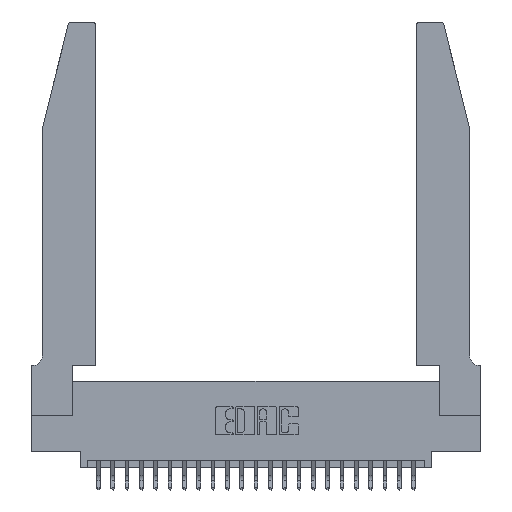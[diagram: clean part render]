
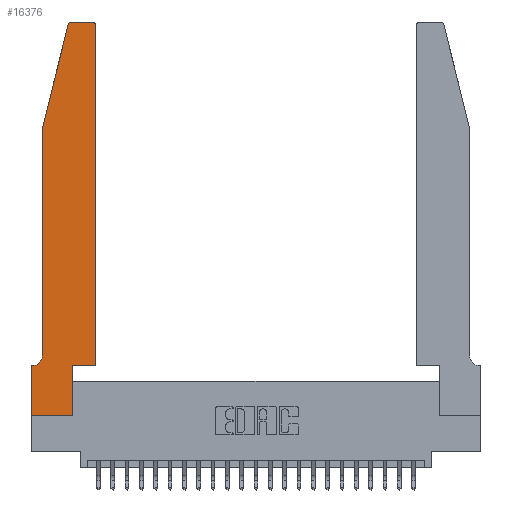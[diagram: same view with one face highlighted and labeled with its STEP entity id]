
A CAD part, top view. The second image highlights one B-rep face of the part: STEP entity #16376.
In plain terms, the highlighted planar face has unit normal (0, 0, 1).
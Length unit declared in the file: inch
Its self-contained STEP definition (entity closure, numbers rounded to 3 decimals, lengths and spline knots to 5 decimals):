
#189 = ORIENTED_EDGE ( 'NONE', *, *, #2360, .T. ) ;
#494 = DIRECTION ( 'NONE',  ( 1., 0., 0. ) ) ;
#630 = LINE ( 'NONE', #22054, #24865 ) ;
#777 = CIRCLE ( 'NONE', #3475, 0.03 ) ;
#1740 = PLANE ( 'NONE',  #3651 ) ;
#1956 = ORIENTED_EDGE ( 'NONE', *, *, #23945, .T. ) ;
#2167 = ORIENTED_EDGE ( 'NONE', *, *, #21607, .T. ) ;
#2360 = EDGE_CURVE ( 'NONE', #24390, #8492, #25150, .T. ) ;
#2530 = LINE ( 'NONE', #25444, #24893 ) ;
#3196 = ORIENTED_EDGE ( 'NONE', *, *, #23025, .T. ) ;
#3216 = DIRECTION ( 'NONE',  ( -1., 0., 0. ) ) ;
#3218 = CARTESIAN_POINT ( 'NONE',  ( 0.0055, 0.35, 0.37 ) ) ;
#3454 = CARTESIAN_POINT ( 'NONE',  ( 0., 0., 0.37 ) ) ;
#3475 = AXIS2_PLACEMENT_3D ( 'NONE', #18984, #17224, #25149 ) ;
#3501 = LINE ( 'NONE', #3454, #16525 ) ;
#3575 = EDGE_LOOP ( 'NONE', ( #5373, #11922, #1956, #13291, #189, #2167, #12911, #5540, #16597, #3196, #10470, #24929 ) ) ;
#3651 = AXIS2_PLACEMENT_3D ( 'NONE', #3890, #12342, #494 ) ;
#3740 = VECTOR ( 'NONE', #5980, 39.37008 ) ;
#3890 = CARTESIAN_POINT ( 'NONE',  ( 0., 0.35, 0.37 ) ) ;
#4422 = DIRECTION ( 'NONE',  ( -1., 0., 0. ) ) ;
#4935 = EDGE_CURVE ( 'NONE', #20659, #11247, #25615, .T. ) ;
#4938 = CARTESIAN_POINT ( 'NONE',  ( 0.284, 2.72, 0.37 ) ) ;
#5136 = VECTOR ( 'NONE', #3216, 39.37008 ) ;
#5190 = CARTESIAN_POINT ( 'NONE',  ( 0.0755, 2., 0.37 ) ) ;
#5373 = ORIENTED_EDGE ( 'NONE', *, *, #4935, .T. ) ;
#5540 = ORIENTED_EDGE ( 'NONE', *, *, #24518, .T. ) ;
#5677 = CARTESIAN_POINT ( 'NONE',  ( 0.25487, 2.72718, 0.37 ) ) ;
#5772 = CARTESIAN_POINT ( 'NONE',  ( 0.4505, 0.35, 0.37 ) ) ;
#5960 = DIRECTION ( 'NONE',  ( 1., 0., 0. ) ) ;
#5980 = DIRECTION ( 'NONE',  ( 0., 1., 0. ) ) ;
#6616 = CARTESIAN_POINT ( 'NONE',  ( 0.0055, 0.42, 0.37 ) ) ;
#6850 = VECTOR ( 'NONE', #20127, 39.37008 ) ;
#7548 = DIRECTION ( 'NONE',  ( -0.239, -0.971, 0. ) ) ;
#8492 = VERTEX_POINT ( 'NONE', #3218 ) ;
#9051 = VERTEX_POINT ( 'NONE', #5677 ) ;
#9086 = LINE ( 'NONE', #22399, #25233 ) ;
#9569 = FACE_OUTER_BOUND ( 'NONE', #3575, .T. ) ;
#9613 = CARTESIAN_POINT ( 'NONE',  ( 0.2865, 0., 0.37 ) ) ;
#10096 = DIRECTION ( 'NONE',  ( 0., 1., 0. ) ) ;
#10343 = VERTEX_POINT ( 'NONE', #9613 ) ;
#10346 = DIRECTION ( 'NONE',  ( 1., 0., 0. ) ) ;
#10423 = AXIS2_PLACEMENT_3D ( 'NONE', #6616, #20361, #4422 ) ;
#10454 = CARTESIAN_POINT ( 'NONE',  ( 0.0755, 0.35, 0.37 ) ) ;
#10470 = ORIENTED_EDGE ( 'NONE', *, *, #21304, .T. ) ;
#10614 = CARTESIAN_POINT ( 'NONE',  ( 0.0755, 2., 0.37 ) ) ;
#11247 = VERTEX_POINT ( 'NONE', #11436 ) ;
#11436 = CARTESIAN_POINT ( 'NONE',  ( 0.284, 2.75, 0.37 ) ) ;
#11484 = LINE ( 'NONE', #17834, #3740 ) ;
#11818 = AXIS2_PLACEMENT_3D ( 'NONE', #4938, #13030, #18896 ) ;
#11922 = ORIENTED_EDGE ( 'NONE', *, *, #21630, .T. ) ;
#12044 = LINE ( 'NONE', #10614, #6850 ) ;
#12342 = DIRECTION ( 'NONE',  ( 0., 0., 1. ) ) ;
#12807 = CARTESIAN_POINT ( 'NONE',  ( 0.2605, 2.75, 0.37 ) ) ;
#12911 = ORIENTED_EDGE ( 'NONE', *, *, #22553, .T. ) ;
#13030 = DIRECTION ( 'NONE',  ( 0., 0., 1. ) ) ;
#13127 = DIRECTION ( 'NONE',  ( 0., -1., 0. ) ) ;
#13291 = ORIENTED_EDGE ( 'NONE', *, *, #15593, .T. ) ;
#13425 = CARTESIAN_POINT ( 'NONE',  ( 0.2865, 0.35, 0.37 ) ) ;
#13945 = EDGE_CURVE ( 'NONE', #20660, #20659, #777, .T. ) ;
#13965 = CIRCLE ( 'NONE', #11818, 0.03 ) ;
#15593 = EDGE_CURVE ( 'NONE', #15837, #24390, #12044, .T. ) ;
#15837 = VERTEX_POINT ( 'NONE', #5190 ) ;
#16081 = VERTEX_POINT ( 'NONE', #5772 ) ;
#16376 = ADVANCED_FACE ( 'NONE', ( #9569 ), #1740, .T. ) ;
#16525 = VECTOR ( 'NONE', #13127, 39.37008 ) ;
#16597 = ORIENTED_EDGE ( 'NONE', *, *, #24557, .T. ) ;
#17224 = DIRECTION ( 'NONE',  ( 0., 0., 1. ) ) ;
#17834 = CARTESIAN_POINT ( 'NONE',  ( 0.4505, 0.35, 0.37 ) ) ;
#18896 = DIRECTION ( 'NONE',  ( 1., 0., 0. ) ) ;
#18984 = CARTESIAN_POINT ( 'NONE',  ( 0.4205, 2.72, 0.37 ) ) ;
#20127 = DIRECTION ( 'NONE',  ( 0., -1., 0. ) ) ;
#20361 = DIRECTION ( 'NONE',  ( 0., 0., -1. ) ) ;
#20478 = VERTEX_POINT ( 'NONE', #21208 ) ;
#20659 = VERTEX_POINT ( 'NONE', #21619 ) ;
#20660 = VERTEX_POINT ( 'NONE', #23518 ) ;
#21053 = CARTESIAN_POINT ( 'NONE',  ( 0.0755, 0.42, 0.37 ) ) ;
#21208 = CARTESIAN_POINT ( 'NONE',  ( 0., 0.35, 0.37 ) ) ;
#21226 = CARTESIAN_POINT ( 'NONE',  ( 0., 0., 0.37 ) ) ;
#21304 = EDGE_CURVE ( 'NONE', #16081, #20660, #11484, .T. ) ;
#21607 = EDGE_CURVE ( 'NONE', #8492, #20478, #24181, .T. ) ;
#21619 = CARTESIAN_POINT ( 'NONE',  ( 0.4205, 2.75, 0.37 ) ) ;
#21630 = EDGE_CURVE ( 'NONE', #11247, #9051, #13965, .T. ) ;
#21788 = VERTEX_POINT ( 'NONE', #21226 ) ;
#21979 = CARTESIAN_POINT ( 'NONE',  ( 0.2865, 0.35, 0.37 ) ) ;
#22019 = LINE ( 'NONE', #21979, #25486 ) ;
#22054 = CARTESIAN_POINT ( 'NONE',  ( 0., 0., 0.37 ) ) ;
#22249 = VERTEX_POINT ( 'NONE', #13425 ) ;
#22399 = CARTESIAN_POINT ( 'NONE',  ( 0.4505, 0.35, 0.37 ) ) ;
#22553 = EDGE_CURVE ( 'NONE', #20478, #21788, #3501, .T. ) ;
#23025 = EDGE_CURVE ( 'NONE', #22249, #16081, #9086, .T. ) ;
#23518 = CARTESIAN_POINT ( 'NONE',  ( 0.4505, 2.72, 0.37 ) ) ;
#23945 = EDGE_CURVE ( 'NONE', #9051, #15837, #2530, .T. ) ;
#24132 = VECTOR ( 'NONE', #24339, 39.37008 ) ;
#24181 = LINE ( 'NONE', #10454, #24132 ) ;
#24339 = DIRECTION ( 'NONE',  ( -1., 0., 0. ) ) ;
#24390 = VERTEX_POINT ( 'NONE', #21053 ) ;
#24518 = EDGE_CURVE ( 'NONE', #21788, #10343, #630, .T. ) ;
#24557 = EDGE_CURVE ( 'NONE', #10343, #22249, #22019, .T. ) ;
#24865 = VECTOR ( 'NONE', #5960, 39.37008 ) ;
#24893 = VECTOR ( 'NONE', #7548, 39.37008 ) ;
#24929 = ORIENTED_EDGE ( 'NONE', *, *, #13945, .T. ) ;
#25149 = DIRECTION ( 'NONE',  ( 1., 0., 0. ) ) ;
#25150 = CIRCLE ( 'NONE', #10423, 0.07 ) ;
#25233 = VECTOR ( 'NONE', #10346, 39.37008 ) ;
#25444 = CARTESIAN_POINT ( 'NONE',  ( 0.0755, 2., 0.37 ) ) ;
#25486 = VECTOR ( 'NONE', #10096, 39.37008 ) ;
#25615 = LINE ( 'NONE', #12807, #5136 ) ;
